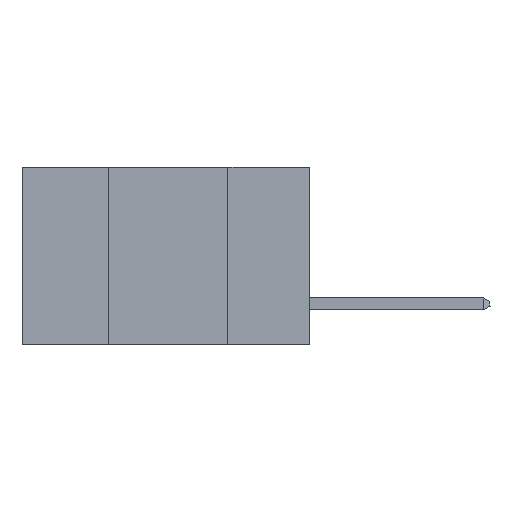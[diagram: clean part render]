
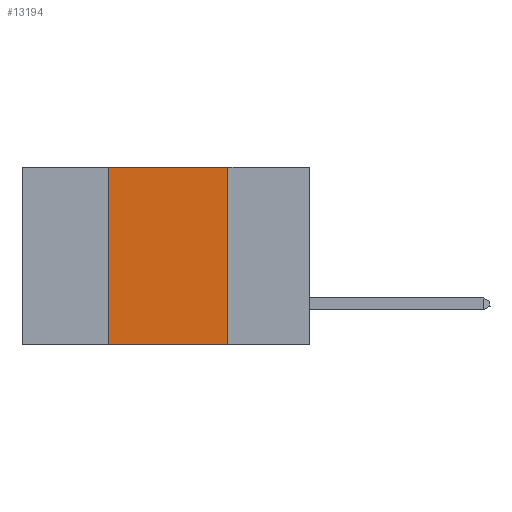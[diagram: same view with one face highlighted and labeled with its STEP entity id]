
A CAD part, left-side view. The second image highlights one B-rep face of the part: STEP entity #13194.
In plain terms, the highlighted planar face has unit normal (-1, 0, 0).
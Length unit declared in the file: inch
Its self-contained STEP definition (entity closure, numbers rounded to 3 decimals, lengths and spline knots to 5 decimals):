
#351 = EDGE_CURVE ( 'NONE', #42891, #9645, #5266, .T. ) ;
#1804 = LINE ( 'NONE', #8167, #26216 ) ;
#3273 = EDGE_CURVE ( 'NONE', #8699, #42891, #8914, .T. ) ;
#5266 = LINE ( 'NONE', #32935, #41854 ) ;
#8167 = CARTESIAN_POINT ( 'NONE',  ( 0., 0.17, 0. ) ) ;
#8699 = VERTEX_POINT ( 'NONE', #23548 ) ;
#8914 = LINE ( 'NONE', #9908, #20571 ) ;
#9437 = ORIENTED_EDGE ( 'NONE', *, *, #351, .F. ) ;
#9645 = VERTEX_POINT ( 'NONE', #11038 ) ;
#9908 = CARTESIAN_POINT ( 'NONE',  ( 0., 0.42, 0. ) ) ;
#11038 = CARTESIAN_POINT ( 'NONE',  ( 0., 0.17, 0. ) ) ;
#11830 = VECTOR ( 'NONE', #16731, 39.37008 ) ;
#13194 = ADVANCED_FACE ( 'NONE', ( #31860 ), #44651, .F. ) ;
#16731 = DIRECTION ( 'NONE',  ( 0., -1., 0. ) ) ;
#19116 = ORIENTED_EDGE ( 'NONE', *, *, #3273, .F. ) ;
#19867 = ORIENTED_EDGE ( 'NONE', *, *, #39652, .F. ) ;
#20571 = VECTOR ( 'NONE', #42093, 39.37008 ) ;
#21100 = VERTEX_POINT ( 'NONE', #42924 ) ;
#23056 = DIRECTION ( 'NONE',  ( 0., -1., 0. ) ) ;
#23548 = CARTESIAN_POINT ( 'NONE',  ( 0., 0.42, -0.37 ) ) ;
#24440 = CARTESIAN_POINT ( 'NONE',  ( 0., 0.6, -0.37 ) ) ;
#26216 = VECTOR ( 'NONE', #39905, 39.37008 ) ;
#26825 = EDGE_CURVE ( 'NONE', #8699, #21100, #30096, .T. ) ;
#27178 = CARTESIAN_POINT ( 'NONE',  ( 0., 0.42, 0. ) ) ;
#30096 = LINE ( 'NONE', #24440, #11830 ) ;
#30554 = CARTESIAN_POINT ( 'NONE',  ( 0., 0.6, 0. ) ) ;
#31000 = DIRECTION ( 'NONE',  ( 1., 0., 0. ) ) ;
#31860 = FACE_OUTER_BOUND ( 'NONE', #39642, .T. ) ;
#32600 = AXIS2_PLACEMENT_3D ( 'NONE', #30554, #31000, #34551 ) ;
#32935 = CARTESIAN_POINT ( 'NONE',  ( 0., 0.6, 0. ) ) ;
#34551 = DIRECTION ( 'NONE',  ( 0., 0., -1. ) ) ;
#39642 = EDGE_LOOP ( 'NONE', ( #19867, #9437, #19116, #41147 ) ) ;
#39652 = EDGE_CURVE ( 'NONE', #9645, #21100, #1804, .T. ) ;
#39905 = DIRECTION ( 'NONE',  ( 0., 0., -1. ) ) ;
#41147 = ORIENTED_EDGE ( 'NONE', *, *, #26825, .T. ) ;
#41854 = VECTOR ( 'NONE', #23056, 39.37008 ) ;
#42093 = DIRECTION ( 'NONE',  ( 0., 0., 1. ) ) ;
#42891 = VERTEX_POINT ( 'NONE', #27178 ) ;
#42924 = CARTESIAN_POINT ( 'NONE',  ( 0., 0.17, -0.37 ) ) ;
#44651 = PLANE ( 'NONE',  #32600 ) ;
